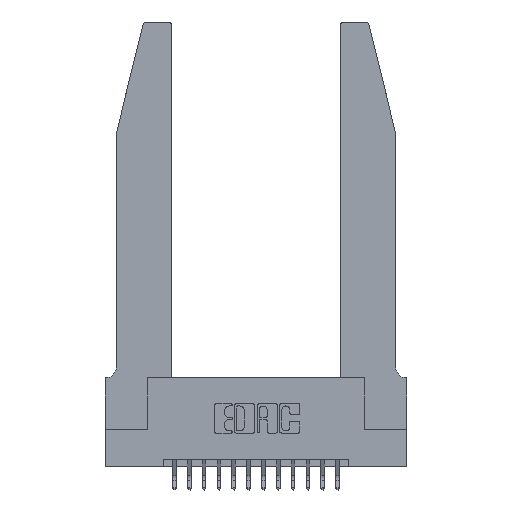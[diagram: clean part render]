
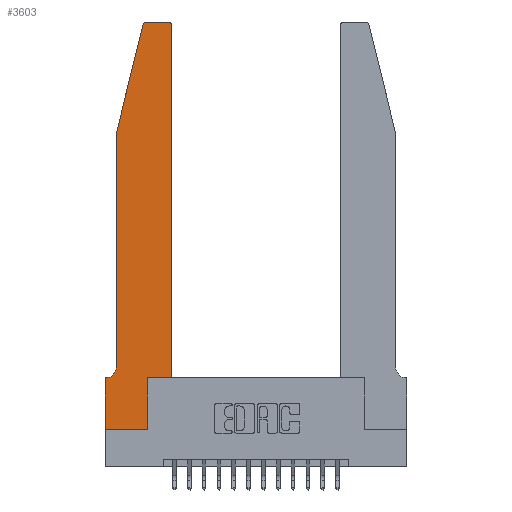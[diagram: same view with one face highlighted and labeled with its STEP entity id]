
A CAD part, top view. The second image highlights one B-rep face of the part: STEP entity #3603.
In plain terms, the highlighted planar face has unit normal (0, 0, 1).
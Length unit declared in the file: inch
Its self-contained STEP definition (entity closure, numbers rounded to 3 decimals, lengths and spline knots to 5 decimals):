
#45 = VERTEX_POINT ( 'NONE', #15874 ) ;
#219 = CARTESIAN_POINT ( 'NONE',  ( 0.4505, 2.72, 0.37 ) ) ;
#701 = FACE_OUTER_BOUND ( 'NONE', #5476, .T. ) ;
#1197 = CARTESIAN_POINT ( 'NONE',  ( 0.0755, 0.42, 0.37 ) ) ;
#1392 = VECTOR ( 'NONE', #13935, 39.37008 ) ;
#1403 = ORIENTED_EDGE ( 'NONE', *, *, #15970, .T. ) ;
#1632 = CARTESIAN_POINT ( 'NONE',  ( 0.0055, 0.35, 0.37 ) ) ;
#1659 = VERTEX_POINT ( 'NONE', #12380 ) ;
#1674 = VECTOR ( 'NONE', #9640, 39.37008 ) ;
#2008 = ORIENTED_EDGE ( 'NONE', *, *, #13563, .T. ) ;
#2058 = CARTESIAN_POINT ( 'NONE',  ( 0.284, 2.75, 0.37 ) ) ;
#2143 = CARTESIAN_POINT ( 'NONE',  ( 0.25487, 2.72718, 0.37 ) ) ;
#2479 = CARTESIAN_POINT ( 'NONE',  ( 0.0755, 2., 0.37 ) ) ;
#2669 = EDGE_CURVE ( 'NONE', #4241, #12295, #17640, .T. ) ;
#3047 = EDGE_CURVE ( 'NONE', #8632, #4241, #10293, .T. ) ;
#3163 = ORIENTED_EDGE ( 'NONE', *, *, #3047, .T. ) ;
#3275 = VECTOR ( 'NONE', #13908, 39.37008 ) ;
#3372 = DIRECTION ( 'NONE',  ( 0., 1., 0. ) ) ;
#3545 = CARTESIAN_POINT ( 'NONE',  ( 0.2865, 0.35, 0.37 ) ) ;
#3603 = ADVANCED_FACE ( 'NONE', ( #701 ), #12447, .T. ) ;
#3659 = DIRECTION ( 'NONE',  ( 0., 0., 1. ) ) ;
#3845 = ORIENTED_EDGE ( 'NONE', *, *, #17819, .T. ) ;
#3882 = CARTESIAN_POINT ( 'NONE',  ( 0., 0., 0.37 ) ) ;
#3943 = CARTESIAN_POINT ( 'NONE',  ( 0., 0.35, 0.37 ) ) ;
#4241 = VERTEX_POINT ( 'NONE', #2143 ) ;
#4362 = LINE ( 'NONE', #2479, #5720 ) ;
#4848 = CARTESIAN_POINT ( 'NONE',  ( 0.0055, 0.42, 0.37 ) ) ;
#5028 = LINE ( 'NONE', #3882, #3275 ) ;
#5319 = CARTESIAN_POINT ( 'NONE',  ( 0.0755, 2., 0.37 ) ) ;
#5476 = EDGE_LOOP ( 'NONE', ( #6346, #3163, #8775, #3845, #12856, #14612, #11964, #12702, #2008, #10780, #1403, #6431 ) ) ;
#5477 = LINE ( 'NONE', #10921, #13509 ) ;
#5702 = VERTEX_POINT ( 'NONE', #15178 ) ;
#5720 = VECTOR ( 'NONE', #10850, 39.37008 ) ;
#6160 = AXIS2_PLACEMENT_3D ( 'NONE', #6230, #13146, #10262 ) ;
#6230 = CARTESIAN_POINT ( 'NONE',  ( 0.4205, 2.72, 0.37 ) ) ;
#6346 = ORIENTED_EDGE ( 'NONE', *, *, #13648, .T. ) ;
#6431 = ORIENTED_EDGE ( 'NONE', *, *, #15449, .T. ) ;
#6578 = DIRECTION ( 'NONE',  ( 1., 0., 0. ) ) ;
#6609 = LINE ( 'NONE', #15305, #13290 ) ;
#6799 = EDGE_CURVE ( 'NONE', #16484, #45, #6609, .T. ) ;
#6820 = EDGE_CURVE ( 'NONE', #15714, #5702, #5028, .T. ) ;
#6826 = VECTOR ( 'NONE', #3372, 39.37008 ) ;
#7104 = CARTESIAN_POINT ( 'NONE',  ( 0.2865, 0.35, 0.37 ) ) ;
#8063 = VERTEX_POINT ( 'NONE', #14071 ) ;
#8373 = LINE ( 'NONE', #7104, #6826 ) ;
#8632 = VERTEX_POINT ( 'NONE', #2058 ) ;
#8775 = ORIENTED_EDGE ( 'NONE', *, *, #2669, .T. ) ;
#9074 = CARTESIAN_POINT ( 'NONE',  ( 0., 0., 0.37 ) ) ;
#9335 = DIRECTION ( 'NONE',  ( 0., 0., 1. ) ) ;
#9601 = EDGE_CURVE ( 'NONE', #10958, #16484, #9826, .T. ) ;
#9640 = DIRECTION ( 'NONE',  ( 0., -1., 0. ) ) ;
#9775 = LINE ( 'NONE', #10952, #17323 ) ;
#9826 = CIRCLE ( 'NONE', #10753, 0.07 ) ;
#10262 = DIRECTION ( 'NONE',  ( 1., 0., 0. ) ) ;
#10293 = CIRCLE ( 'NONE', #18444, 0.03 ) ;
#10580 = DIRECTION ( 'NONE',  ( 0., 0., -1. ) ) ;
#10753 = AXIS2_PLACEMENT_3D ( 'NONE', #4848, #10580, #17653 ) ;
#10780 = ORIENTED_EDGE ( 'NONE', *, *, #12780, .T. ) ;
#10850 = DIRECTION ( 'NONE',  ( 0., -1., 0. ) ) ;
#10921 = CARTESIAN_POINT ( 'NONE',  ( 0.4505, 0.35, 0.37 ) ) ;
#10952 = CARTESIAN_POINT ( 'NONE',  ( 0.4505, 0.35, 0.37 ) ) ;
#10958 = VERTEX_POINT ( 'NONE', #1197 ) ;
#11964 = ORIENTED_EDGE ( 'NONE', *, *, #18285, .T. ) ;
#12223 = CARTESIAN_POINT ( 'NONE',  ( 0.284, 2.72, 0.37 ) ) ;
#12295 = VERTEX_POINT ( 'NONE', #12516 ) ;
#12380 = CARTESIAN_POINT ( 'NONE',  ( 0.4505, 0.35, 0.37 ) ) ;
#12447 = PLANE ( 'NONE',  #16522 ) ;
#12516 = CARTESIAN_POINT ( 'NONE',  ( 0.0755, 2., 0.37 ) ) ;
#12606 = VERTEX_POINT ( 'NONE', #3545 ) ;
#12702 = ORIENTED_EDGE ( 'NONE', *, *, #6820, .T. ) ;
#12780 = EDGE_CURVE ( 'NONE', #12606, #1659, #5477, .T. ) ;
#12856 = ORIENTED_EDGE ( 'NONE', *, *, #9601, .T. ) ;
#13146 = DIRECTION ( 'NONE',  ( 0., 0., 1. ) ) ;
#13290 = VECTOR ( 'NONE', #18168, 39.37008 ) ;
#13509 = VECTOR ( 'NONE', #18324, 39.37008 ) ;
#13563 = EDGE_CURVE ( 'NONE', #5702, #12606, #8373, .T. ) ;
#13648 = EDGE_CURVE ( 'NONE', #8063, #8632, #16378, .T. ) ;
#13908 = DIRECTION ( 'NONE',  ( 1., 0., 0. ) ) ;
#13935 = DIRECTION ( 'NONE',  ( -0.239, -0.971, 0. ) ) ;
#13943 = LINE ( 'NONE', #16664, #1674 ) ;
#14071 = CARTESIAN_POINT ( 'NONE',  ( 0.4205, 2.75, 0.37 ) ) ;
#14606 = VECTOR ( 'NONE', #16092, 39.37008 ) ;
#14612 = ORIENTED_EDGE ( 'NONE', *, *, #6799, .T. ) ;
#15178 = CARTESIAN_POINT ( 'NONE',  ( 0.2865, 0., 0.37 ) ) ;
#15305 = CARTESIAN_POINT ( 'NONE',  ( 0.0755, 0.35, 0.37 ) ) ;
#15449 = EDGE_CURVE ( 'NONE', #17259, #8063, #16901, .T. ) ;
#15714 = VERTEX_POINT ( 'NONE', #9074 ) ;
#15874 = CARTESIAN_POINT ( 'NONE',  ( 0., 0.35, 0.37 ) ) ;
#15970 = EDGE_CURVE ( 'NONE', #1659, #17259, #9775, .T. ) ;
#15972 = DIRECTION ( 'NONE',  ( 0., 1., 0. ) ) ;
#16092 = DIRECTION ( 'NONE',  ( -1., 0., 0. ) ) ;
#16378 = LINE ( 'NONE', #17462, #14606 ) ;
#16484 = VERTEX_POINT ( 'NONE', #1632 ) ;
#16487 = DIRECTION ( 'NONE',  ( 1., 0., 0. ) ) ;
#16522 = AXIS2_PLACEMENT_3D ( 'NONE', #3943, #9335, #16487 ) ;
#16664 = CARTESIAN_POINT ( 'NONE',  ( 0., 0., 0.37 ) ) ;
#16901 = CIRCLE ( 'NONE', #6160, 0.03 ) ;
#17259 = VERTEX_POINT ( 'NONE', #219 ) ;
#17323 = VECTOR ( 'NONE', #15972, 39.37008 ) ;
#17462 = CARTESIAN_POINT ( 'NONE',  ( 0.2605, 2.75, 0.37 ) ) ;
#17640 = LINE ( 'NONE', #5319, #1392 ) ;
#17653 = DIRECTION ( 'NONE',  ( -1., 0., 0. ) ) ;
#17819 = EDGE_CURVE ( 'NONE', #12295, #10958, #4362, .T. ) ;
#18168 = DIRECTION ( 'NONE',  ( -1., 0., 0. ) ) ;
#18285 = EDGE_CURVE ( 'NONE', #45, #15714, #13943, .T. ) ;
#18324 = DIRECTION ( 'NONE',  ( 1., 0., 0. ) ) ;
#18444 = AXIS2_PLACEMENT_3D ( 'NONE', #12223, #3659, #6578 ) ;
